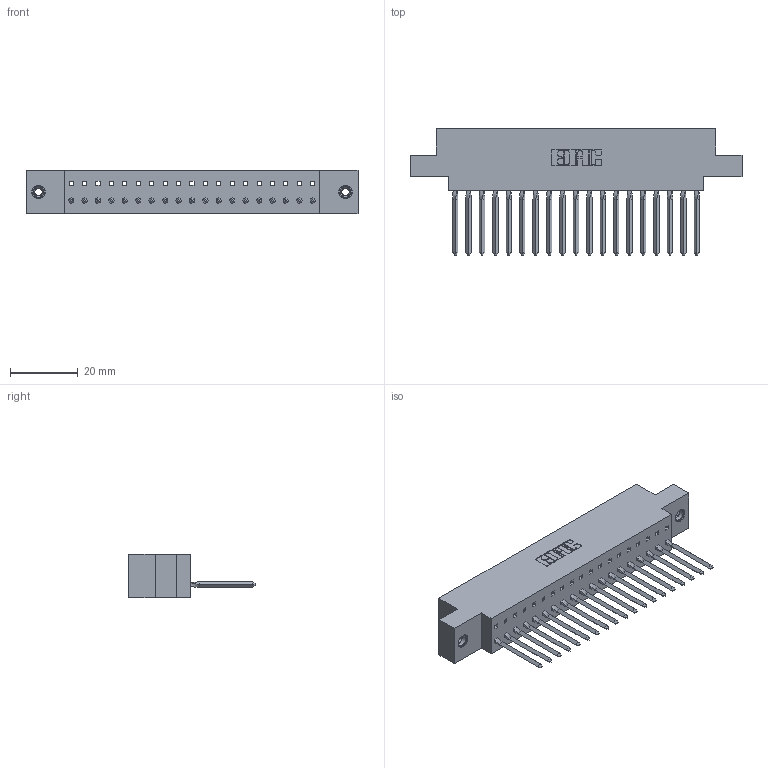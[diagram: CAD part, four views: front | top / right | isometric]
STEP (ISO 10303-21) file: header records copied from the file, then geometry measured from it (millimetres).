
FILE_DESCRIPTION (( 'STEP AP203' ), '1' );
FILE_NAME ('317-019-542-678.STEP', '2020-02-27T16:20:20', ( '' ), ( '' ), 'SwSTEP 2.0', 'SolidWorks 2016', '' );
FILE_SCHEMA (( 'CONFIG_CONTROL_DESIGN' ));
Length unit declared in the file: inch
Products named in the file (4): 317-019-542-678; 317-290-003_542; 345-250-001_345-250-003-102; 317 Part_.156 Dia - TI
Assembly tree (22 placements, depth 2):
  317-019-542-678
    317 Part_.156 Dia - TI
    317-290-003_542  x19
    345-250-001_345-250-003-102  x2
Bounding box: 97.99 x 37.34 x 12.7 mm (x, y, z)
Volume: 14519.2 mm3; surface area: 17219.6 mm2
Topology: 22 solids, 22 shells, 1587 faces, 4534 edges, 2926 vertices
Faces by surface type: plane 1306, cylinder 189, bspline 76, cone 12, torus 4
Entity records: 30268 total; most frequent: CARTESIAN_POINT 5585, ORIENTED_EDGE 5260, DIRECTION 4466, EDGE_CURVE 2630, LINE 2440, VECTOR 2440, VERTEX_POINT 1744, AXIS2_PLACEMENT_3D 1013
